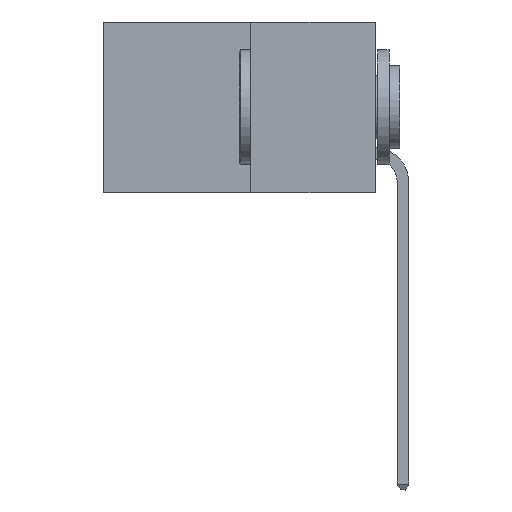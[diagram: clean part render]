
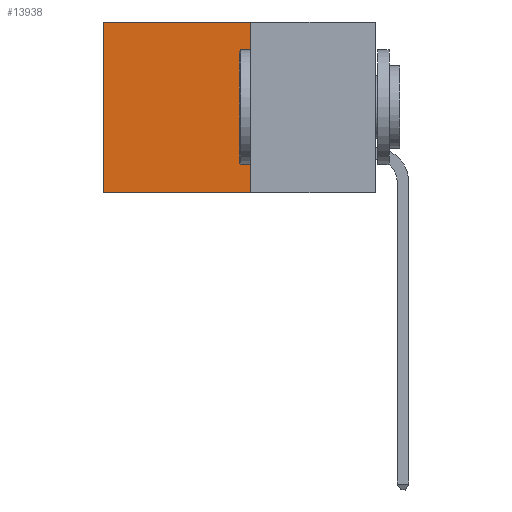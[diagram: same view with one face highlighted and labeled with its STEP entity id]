
A CAD part, left-side view. The second image highlights one B-rep face of the part: STEP entity #13938.
In plain terms, the highlighted planar face has unit normal (-1, 0, 0).
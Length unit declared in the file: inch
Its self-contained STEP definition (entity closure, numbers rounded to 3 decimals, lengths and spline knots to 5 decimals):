
#2418 = VERTEX_POINT ( 'NONE', #15052 ) ;
#3102 = VECTOR ( 'NONE', #5447, 39.37008 ) ;
#3276 = EDGE_CURVE ( 'NONE', #9022, #8504, #17235, .T. ) ;
#3471 = CARTESIAN_POINT ( 'NONE',  ( 0.277, 0.59, 0. ) ) ;
#3848 = DIRECTION ( 'NONE',  ( 0., 1., 0. ) ) ;
#4605 = PLANE ( 'NONE',  #13477 ) ;
#5447 = DIRECTION ( 'NONE',  ( 0., 0., -1. ) ) ;
#5568 = ORIENTED_EDGE ( 'NONE', *, *, #16385, .F. ) ;
#5795 = ORIENTED_EDGE ( 'NONE', *, *, #10994, .T. ) ;
#5873 = ORIENTED_EDGE ( 'NONE', *, *, #11623, .F. ) ;
#6005 = CARTESIAN_POINT ( 'NONE',  ( 0.277, 0.27, -0.37 ) ) ;
#6517 = DIRECTION ( 'NONE',  ( 0., 1., 0. ) ) ;
#7409 = DIRECTION ( 'NONE',  ( 0., 0., -1. ) ) ;
#7445 = VECTOR ( 'NONE', #3848, 39.37008 ) ;
#7854 = LINE ( 'NONE', #14726, #7445 ) ;
#7891 = CARTESIAN_POINT ( 'NONE',  ( 0.277, 0.27, 0. ) ) ;
#8425 = CARTESIAN_POINT ( 'NONE',  ( 0.277, 0.59, -0.37 ) ) ;
#8504 = VERTEX_POINT ( 'NONE', #3471 ) ;
#8715 = CARTESIAN_POINT ( 'NONE',  ( 0.277, 0.27, 0. ) ) ;
#9022 = VERTEX_POINT ( 'NONE', #8715 ) ;
#9220 = CARTESIAN_POINT ( 'NONE',  ( 0.277, 0.59, -0.37 ) ) ;
#10470 = VECTOR ( 'NONE', #13305, 39.37008 ) ;
#10994 = EDGE_CURVE ( 'NONE', #8504, #13764, #14031, .T. ) ;
#11623 = EDGE_CURVE ( 'NONE', #2418, #13764, #7854, .T. ) ;
#12682 = EDGE_LOOP ( 'NONE', ( #5795, #5873, #5568, #14926 ) ) ;
#12869 = FACE_OUTER_BOUND ( 'NONE', #12682, .T. ) ;
#13305 = DIRECTION ( 'NONE',  ( 0., 0., -1. ) ) ;
#13477 = AXIS2_PLACEMENT_3D ( 'NONE', #6005, #15450, #7409 ) ;
#13586 = LINE ( 'NONE', #17577, #3102 ) ;
#13749 = VECTOR ( 'NONE', #6517, 39.37008 ) ;
#13764 = VERTEX_POINT ( 'NONE', #8425 ) ;
#13938 = ADVANCED_FACE ( 'NONE', ( #12869 ), #4605, .F. ) ;
#14031 = LINE ( 'NONE', #9220, #10470 ) ;
#14726 = CARTESIAN_POINT ( 'NONE',  ( 0.277, 0.27, -0.37 ) ) ;
#14926 = ORIENTED_EDGE ( 'NONE', *, *, #3276, .T. ) ;
#15052 = CARTESIAN_POINT ( 'NONE',  ( 0.277, 0.27, -0.37 ) ) ;
#15450 = DIRECTION ( 'NONE',  ( 1., 0., 0. ) ) ;
#16385 = EDGE_CURVE ( 'NONE', #9022, #2418, #13586, .T. ) ;
#17235 = LINE ( 'NONE', #7891, #13749 ) ;
#17577 = CARTESIAN_POINT ( 'NONE',  ( 0.277, 0.27, -0.37 ) ) ;
